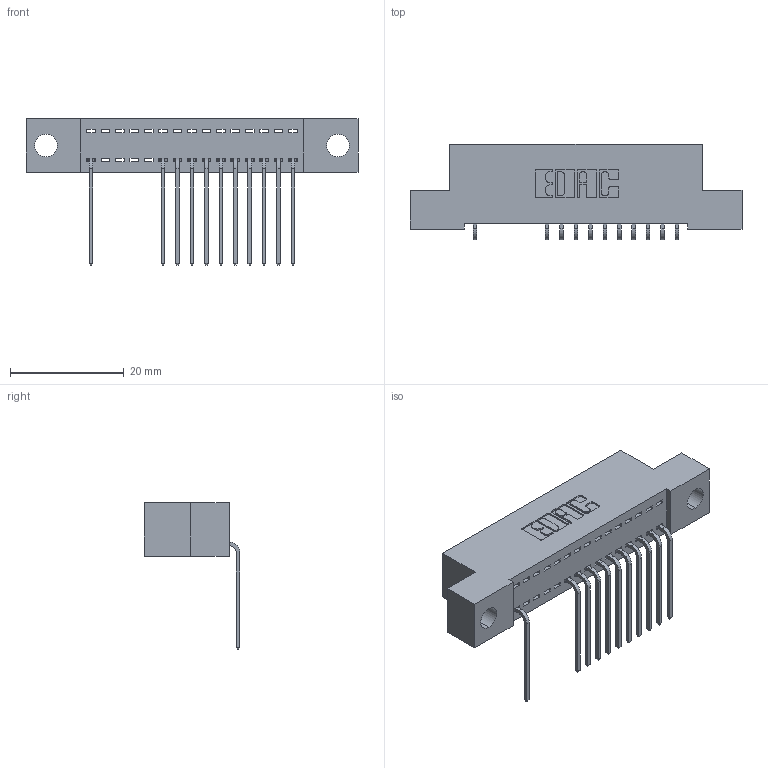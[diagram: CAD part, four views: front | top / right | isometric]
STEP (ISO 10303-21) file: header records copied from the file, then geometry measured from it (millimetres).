
FILE_DESCRIPTION (( 'STEP AP203' ), '1' );
FILE_NAME ('392-015-559-104.STEP', '2018-08-15T01:17:10', ( '' ), ( '' ), 'SwSTEP 2.0', 'SolidWorks 2016', '' );
FILE_SCHEMA (( 'CONFIG_CONTROL_DESIGN' ));
Length unit declared in the file: inch
Products named in the file (3): 345-292-001_558 559 Tail - 1; 392-015-559-104; 342 Part_.156 TH
Assembly tree (12 placements, depth 2):
  392-015-559-104
    342 Part_.156 TH
    345-292-001_558 559 Tail - 1  x11
Bounding box: 58.42 x 16.83 x 25.78 mm (x, y, z)
Volume: 4926.7 mm3; surface area: 6520.4 mm2
Topology: 12 solids, 12 shells, 818 faces, 2469 edges, 1630 vertices
Faces by surface type: plane 598, cylinder 220
Entity records: 12489 total; most frequent: CARTESIAN_POINT 2183, ORIENTED_EDGE 2138, DIRECTION 1891, EDGE_CURVE 1069, VECTOR 941, LINE 941, VERTEX_POINT 710, AXIS2_PLACEMENT_3D 475
